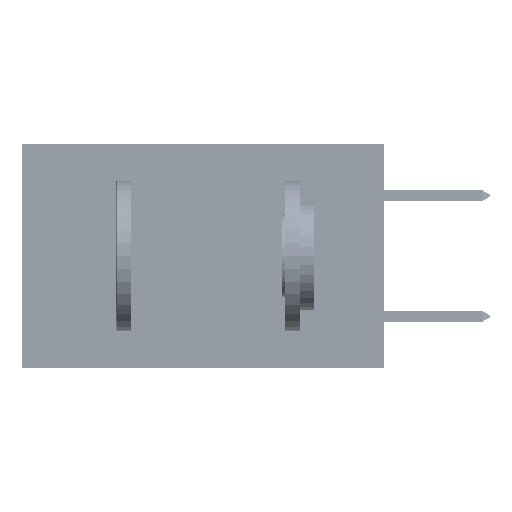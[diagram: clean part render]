
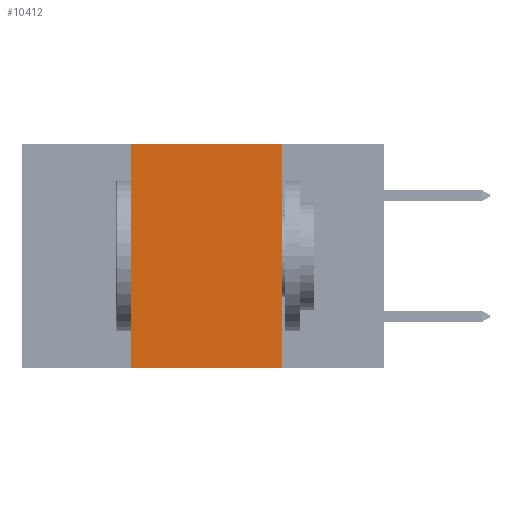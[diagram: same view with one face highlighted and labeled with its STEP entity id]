
A CAD part, left-side view. The second image highlights one B-rep face of the part: STEP entity #10412.
In plain terms, the highlighted planar face has unit normal (-1, 0, 0).
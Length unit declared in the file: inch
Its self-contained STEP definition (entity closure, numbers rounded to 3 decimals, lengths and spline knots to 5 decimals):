
#2414 = EDGE_CURVE ( 'NONE', #38397, #4536, #45232, .T. ) ;
#3493 = EDGE_CURVE ( 'NONE', #7227, #36158, #23645, .T. ) ;
#3833 = ORIENTED_EDGE ( 'NONE', *, *, #3493, .F. ) ;
#4536 = VERTEX_POINT ( 'NONE', #26837 ) ;
#4647 = CARTESIAN_POINT ( 'NONE',  ( 0., 0.6, -0.37 ) ) ;
#5698 = ORIENTED_EDGE ( 'NONE', *, *, #2414, .F. ) ;
#7227 = VERTEX_POINT ( 'NONE', #13113 ) ;
#8814 = DIRECTION ( 'NONE',  ( 0., -1., 0. ) ) ;
#10412 = ADVANCED_FACE ( 'NONE', ( #42760 ), #44396, .F. ) ;
#13099 = CARTESIAN_POINT ( 'NONE',  ( 0., 0.17, 0. ) ) ;
#13113 = CARTESIAN_POINT ( 'NONE',  ( 0., 0.17, 0. ) ) ;
#18021 = DIRECTION ( 'NONE',  ( 0., 0., 1. ) ) ;
#18570 = DIRECTION ( 'NONE',  ( 0., -1., 0. ) ) ;
#19074 = VECTOR ( 'NONE', #8814, 39.37008 ) ;
#19778 = ORIENTED_EDGE ( 'NONE', *, *, #27503, .T. ) ;
#20429 = EDGE_CURVE ( 'NONE', #4536, #7227, #35181, .T. ) ;
#20776 = AXIS2_PLACEMENT_3D ( 'NONE', #21570, #33209, #32715 ) ;
#21570 = CARTESIAN_POINT ( 'NONE',  ( 0., 0.6, 0. ) ) ;
#23645 = LINE ( 'NONE', #13099, #24814 ) ;
#24418 = LINE ( 'NONE', #4647, #19074 ) ;
#24814 = VECTOR ( 'NONE', #39823, 39.37008 ) ;
#26837 = CARTESIAN_POINT ( 'NONE',  ( 0., 0.42, 0. ) ) ;
#27446 = ORIENTED_EDGE ( 'NONE', *, *, #20429, .F. ) ;
#27503 = EDGE_CURVE ( 'NONE', #38397, #36158, #24418, .T. ) ;
#29034 = CARTESIAN_POINT ( 'NONE',  ( 0., 0.42, 0. ) ) ;
#31692 = CARTESIAN_POINT ( 'NONE',  ( 0., 0.17, -0.37 ) ) ;
#32715 = DIRECTION ( 'NONE',  ( 0., 0., -1. ) ) ;
#33104 = CARTESIAN_POINT ( 'NONE',  ( 0., 0.42, -0.37 ) ) ;
#33209 = DIRECTION ( 'NONE',  ( 1., 0., 0. ) ) ;
#35181 = LINE ( 'NONE', #37603, #42955 ) ;
#36158 = VERTEX_POINT ( 'NONE', #31692 ) ;
#37603 = CARTESIAN_POINT ( 'NONE',  ( 0., 0.6, 0. ) ) ;
#38100 = VECTOR ( 'NONE', #18021, 39.37008 ) ;
#38397 = VERTEX_POINT ( 'NONE', #33104 ) ;
#39823 = DIRECTION ( 'NONE',  ( 0., 0., -1. ) ) ;
#42760 = FACE_OUTER_BOUND ( 'NONE', #46223, .T. ) ;
#42955 = VECTOR ( 'NONE', #18570, 39.37008 ) ;
#44396 = PLANE ( 'NONE',  #20776 ) ;
#45232 = LINE ( 'NONE', #29034, #38100 ) ;
#46223 = EDGE_LOOP ( 'NONE', ( #3833, #27446, #5698, #19778 ) ) ;
